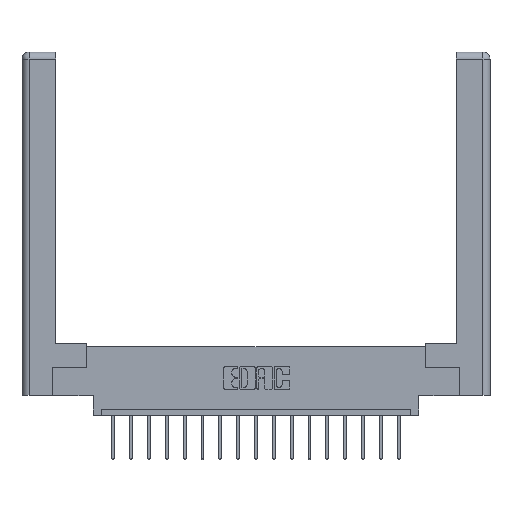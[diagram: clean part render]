
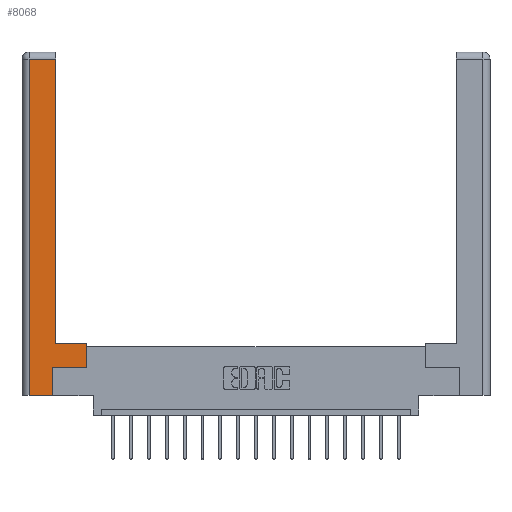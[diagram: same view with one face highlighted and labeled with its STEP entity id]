
A CAD part, top view. The second image highlights one B-rep face of the part: STEP entity #8068.
In plain terms, the highlighted planar face has unit normal (0, 0, 1).
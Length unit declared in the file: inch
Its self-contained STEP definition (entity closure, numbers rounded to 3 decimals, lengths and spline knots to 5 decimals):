
#68 = VECTOR ( 'NONE', #6400, 39.37008 ) ;
#498 = VECTOR ( 'NONE', #8559, 39.37008 ) ;
#785 = ORIENTED_EDGE ( 'NONE', *, *, #6519, .T. ) ;
#1352 = PLANE ( 'NONE',  #10023 ) ;
#1357 = EDGE_CURVE ( 'NONE', #4518, #16172, #7479, .T. ) ;
#1715 = ORIENTED_EDGE ( 'NONE', *, *, #1357, .T. ) ;
#1737 = CARTESIAN_POINT ( 'NONE',  ( 0.0615, 2.94, 0. ) ) ;
#1832 = VERTEX_POINT ( 'NONE', #4647 ) ;
#2198 = DIRECTION ( 'NONE',  ( 1., 0., 0. ) ) ;
#2337 = CARTESIAN_POINT ( 'NONE',  ( 0.295, 3., 0. ) ) ;
#2406 = CARTESIAN_POINT ( 'NONE',  ( 0.265, 0.245, 0. ) ) ;
#2525 = VECTOR ( 'NONE', #11021, 39.37008 ) ;
#2552 = LINE ( 'NONE', #4497, #498 ) ;
#2567 = VECTOR ( 'NONE', #8758, 39.37008 ) ;
#2631 = ORIENTED_EDGE ( 'NONE', *, *, #11243, .T. ) ;
#3210 = CARTESIAN_POINT ( 'NONE',  ( 0.0615, 0., 0. ) ) ;
#3416 = CARTESIAN_POINT ( 'NONE',  ( 0.0615, 2.94, 0. ) ) ;
#3917 = ORIENTED_EDGE ( 'NONE', *, *, #10944, .T. ) ;
#4379 = CARTESIAN_POINT ( 'NONE',  ( 0., 0., 0. ) ) ;
#4442 = VERTEX_POINT ( 'NONE', #7860 ) ;
#4497 = CARTESIAN_POINT ( 'NONE',  ( 0.565, 0.245, 0. ) ) ;
#4518 = VERTEX_POINT ( 'NONE', #1737 ) ;
#4647 = CARTESIAN_POINT ( 'NONE',  ( 0.295, 2.94, 0. ) ) ;
#4805 = CARTESIAN_POINT ( 'NONE',  ( 0.565, 0.45, 0. ) ) ;
#5607 = CARTESIAN_POINT ( 'NONE',  ( 0.0615, 0., 0. ) ) ;
#5802 = DIRECTION ( 'NONE',  ( 0., 0., -1. ) ) ;
#6042 = VERTEX_POINT ( 'NONE', #9999 ) ;
#6306 = LINE ( 'NONE', #2337, #2525 ) ;
#6400 = DIRECTION ( 'NONE',  ( -1., 0., 0. ) ) ;
#6519 = EDGE_CURVE ( 'NONE', #16172, #10168, #8817, .T. ) ;
#6598 = CARTESIAN_POINT ( 'NONE',  ( 0.295, 0.45, 0. ) ) ;
#6654 = EDGE_CURVE ( 'NONE', #1832, #4518, #17420, .T. ) ;
#6738 = CARTESIAN_POINT ( 'NONE',  ( 0.295, 0.45, 0. ) ) ;
#6760 = VECTOR ( 'NONE', #8469, 39.37008 ) ;
#6812 = VECTOR ( 'NONE', #2198, 39.37008 ) ;
#6882 = EDGE_CURVE ( 'NONE', #6042, #4442, #2552, .T. ) ;
#7136 = DIRECTION ( 'NONE',  ( -1., 0., 0. ) ) ;
#7479 = LINE ( 'NONE', #3210, #2567 ) ;
#7860 = CARTESIAN_POINT ( 'NONE',  ( 0.565, 0.245, 0. ) ) ;
#8068 = ADVANCED_FACE ( 'NONE', ( #16564 ), #1352, .F. ) ;
#8154 = ORIENTED_EDGE ( 'NONE', *, *, #15359, .T. ) ;
#8177 = EDGE_CURVE ( 'NONE', #10168, #6042, #12721, .T. ) ;
#8226 = ORIENTED_EDGE ( 'NONE', *, *, #6654, .T. ) ;
#8469 = DIRECTION ( 'NONE',  ( 0., 1., 0. ) ) ;
#8559 = DIRECTION ( 'NONE',  ( 1., 0., 0. ) ) ;
#8758 = DIRECTION ( 'NONE',  ( 0., -1., 0. ) ) ;
#8817 = LINE ( 'NONE', #9332, #6812 ) ;
#9332 = CARTESIAN_POINT ( 'NONE',  ( 0.265, 0., 0. ) ) ;
#9563 = VECTOR ( 'NONE', #16947, 39.37008 ) ;
#9989 = VECTOR ( 'NONE', #15339, 39.37008 ) ;
#9999 = CARTESIAN_POINT ( 'NONE',  ( 0.265, 0.245, 0. ) ) ;
#10023 = AXIS2_PLACEMENT_3D ( 'NONE', #4379, #5802, #7136 ) ;
#10168 = VERTEX_POINT ( 'NONE', #18568 ) ;
#10944 = EDGE_CURVE ( 'NONE', #4442, #11901, #14224, .T. ) ;
#11021 = DIRECTION ( 'NONE',  ( 0., 1., 0. ) ) ;
#11243 = EDGE_CURVE ( 'NONE', #11901, #12500, #17285, .T. ) ;
#11901 = VERTEX_POINT ( 'NONE', #4805 ) ;
#12500 = VERTEX_POINT ( 'NONE', #6598 ) ;
#12721 = LINE ( 'NONE', #2406, #9989 ) ;
#14113 = ORIENTED_EDGE ( 'NONE', *, *, #8177, .T. ) ;
#14224 = LINE ( 'NONE', #18520, #6760 ) ;
#15339 = DIRECTION ( 'NONE',  ( 0., 1., 0. ) ) ;
#15359 = EDGE_CURVE ( 'NONE', #12500, #1832, #6306, .T. ) ;
#16140 = EDGE_LOOP ( 'NONE', ( #8154, #8226, #1715, #785, #14113, #16476, #3917, #2631 ) ) ;
#16172 = VERTEX_POINT ( 'NONE', #5607 ) ;
#16476 = ORIENTED_EDGE ( 'NONE', *, *, #6882, .T. ) ;
#16564 = FACE_OUTER_BOUND ( 'NONE', #16140, .T. ) ;
#16947 = DIRECTION ( 'NONE',  ( -1., 0., 0. ) ) ;
#17285 = LINE ( 'NONE', #6738, #9563 ) ;
#17420 = LINE ( 'NONE', #3416, #68 ) ;
#18520 = CARTESIAN_POINT ( 'NONE',  ( 0.565, 0.45, 0. ) ) ;
#18568 = CARTESIAN_POINT ( 'NONE',  ( 0.265, 0., 0. ) ) ;
